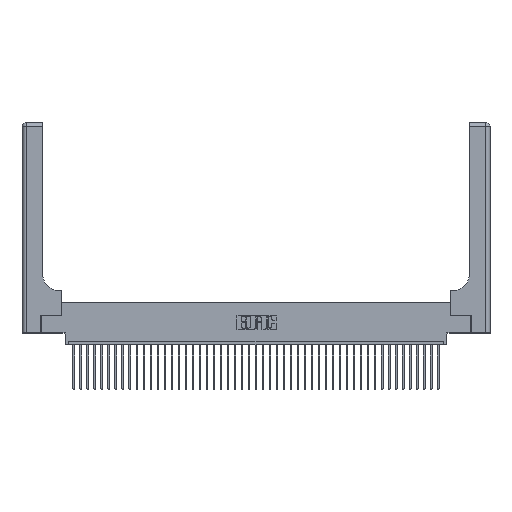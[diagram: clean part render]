
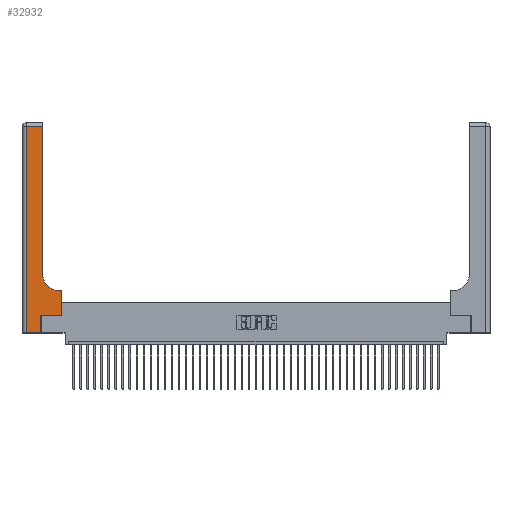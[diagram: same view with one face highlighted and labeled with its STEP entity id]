
A CAD part, top view. The second image highlights one B-rep face of the part: STEP entity #32932.
In plain terms, the highlighted planar face has unit normal (0, 0, 1).
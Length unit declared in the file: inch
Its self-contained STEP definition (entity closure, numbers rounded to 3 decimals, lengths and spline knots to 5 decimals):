
#209 = DIRECTION ( 'NONE',  ( 0., 1., 0. ) ) ;
#854 = EDGE_CURVE ( 'NONE', #1637, #6872, #2060, .T. ) ;
#1092 = CARTESIAN_POINT ( 'NONE',  ( 0., 3., 0.37 ) ) ;
#1114 = CARTESIAN_POINT ( 'NONE',  ( 0.269, 0.25, 0.37 ) ) ;
#1637 = VERTEX_POINT ( 'NONE', #42961 ) ;
#2060 = CIRCLE ( 'NONE', #29750, 0.25 ) ;
#3450 = CARTESIAN_POINT ( 'NONE',  ( 0.269, 0., 0.37 ) ) ;
#3583 = VECTOR ( 'NONE', #209, 39.37008 ) ;
#4726 = VERTEX_POINT ( 'NONE', #15478 ) ;
#5532 = CARTESIAN_POINT ( 'NONE',  ( 0.06, 0., 0.37 ) ) ;
#5651 = ORIENTED_EDGE ( 'NONE', *, *, #35412, .T. ) ;
#6872 = VERTEX_POINT ( 'NONE', #14135 ) ;
#7210 = VECTOR ( 'NONE', #16628, 39.37008 ) ;
#8408 = CARTESIAN_POINT ( 'NONE',  ( 0.5415, 0.85, 0.37 ) ) ;
#9721 = EDGE_LOOP ( 'NONE', ( #29749, #23551, #40036, #22765, #22659, #40509, #21154, #5651, #32038 ) ) ;
#10462 = LINE ( 'NONE', #3450, #27368 ) ;
#11140 = DIRECTION ( 'NONE',  ( -1., 0., 0. ) ) ;
#11336 = VERTEX_POINT ( 'NONE', #41987 ) ;
#11746 = DIRECTION ( 'NONE',  ( -1., 0., 0. ) ) ;
#12365 = CARTESIAN_POINT ( 'NONE',  ( 0.5585, 0.25, 0.37 ) ) ;
#13277 = EDGE_CURVE ( 'NONE', #34375, #34233, #33608, .T. ) ;
#13464 = CARTESIAN_POINT ( 'NONE',  ( 0., 0., 0.37 ) ) ;
#13812 = CARTESIAN_POINT ( 'NONE',  ( 0.2915, 3., 0.37 ) ) ;
#14135 = CARTESIAN_POINT ( 'NONE',  ( 0.2915, 0.85, 0.37 ) ) ;
#14227 = VECTOR ( 'NONE', #23462, 39.37008 ) ;
#15153 = VECTOR ( 'NONE', #26206, 39.37008 ) ;
#15209 = DIRECTION ( 'NONE',  ( 1., 0., 0. ) ) ;
#15478 = CARTESIAN_POINT ( 'NONE',  ( 0.2915, 2.94, 0.37 ) ) ;
#16187 = LINE ( 'NONE', #23809, #7210 ) ;
#16628 = DIRECTION ( 'NONE',  ( 1., 0., 0. ) ) ;
#18072 = VERTEX_POINT ( 'NONE', #1114 ) ;
#18288 = VECTOR ( 'NONE', #33335, 39.37008 ) ;
#18514 = CARTESIAN_POINT ( 'NONE',  ( 0.2915, 0.6, 0.37 ) ) ;
#18700 = EDGE_CURVE ( 'NONE', #6872, #4726, #23651, .T. ) ;
#20914 = CARTESIAN_POINT ( 'NONE',  ( 0.5585, 0.6, 0.37 ) ) ;
#21154 = ORIENTED_EDGE ( 'NONE', *, *, #40688, .T. ) ;
#22008 = DIRECTION ( 'NONE',  ( 0., 0., -1. ) ) ;
#22659 = ORIENTED_EDGE ( 'NONE', *, *, #35820, .T. ) ;
#22765 = ORIENTED_EDGE ( 'NONE', *, *, #34485, .T. ) ;
#23462 = DIRECTION ( 'NONE',  ( 1., 0., 0. ) ) ;
#23551 = ORIENTED_EDGE ( 'NONE', *, *, #40330, .T. ) ;
#23651 = LINE ( 'NONE', #13812, #3583 ) ;
#23809 = CARTESIAN_POINT ( 'NONE',  ( 0.269, 0.25, 0.37 ) ) ;
#24108 = VERTEX_POINT ( 'NONE', #12365 ) ;
#24414 = DIRECTION ( 'NONE',  ( 0., -1., 0. ) ) ;
#26206 = DIRECTION ( 'NONE',  ( 0., 1., 0. ) ) ;
#26987 = CARTESIAN_POINT ( 'NONE',  ( 0., 2.94, 0.37 ) ) ;
#27368 = VECTOR ( 'NONE', #40761, 39.37008 ) ;
#28361 = LINE ( 'NONE', #38571, #15153 ) ;
#28410 = CARTESIAN_POINT ( 'NONE',  ( 0.06, 3., 0.37 ) ) ;
#29533 = LINE ( 'NONE', #18514, #33225 ) ;
#29749 = ORIENTED_EDGE ( 'NONE', *, *, #18700, .T. ) ;
#29750 = AXIS2_PLACEMENT_3D ( 'NONE', #8408, #22008, #15209 ) ;
#30598 = VERTEX_POINT ( 'NONE', #20914 ) ;
#32038 = ORIENTED_EDGE ( 'NONE', *, *, #854, .T. ) ;
#32932 = ADVANCED_FACE ( 'NONE', ( #40286 ), #38118, .F. ) ;
#33225 = VECTOR ( 'NONE', #11746, 39.37008 ) ;
#33335 = DIRECTION ( 'NONE',  ( -1., 0., 0. ) ) ;
#33608 = LINE ( 'NONE', #28410, #35170 ) ;
#34233 = VERTEX_POINT ( 'NONE', #5532 ) ;
#34375 = VERTEX_POINT ( 'NONE', #42677 ) ;
#34485 = EDGE_CURVE ( 'NONE', #34233, #11336, #42220, .T. ) ;
#35170 = VECTOR ( 'NONE', #24414, 39.37008 ) ;
#35203 = DIRECTION ( 'NONE',  ( 0., 0., -1. ) ) ;
#35412 = EDGE_CURVE ( 'NONE', #30598, #1637, #29533, .T. ) ;
#35820 = EDGE_CURVE ( 'NONE', #11336, #18072, #10462, .T. ) ;
#36276 = LINE ( 'NONE', #26987, #18288 ) ;
#38118 = PLANE ( 'NONE',  #39278 ) ;
#38571 = CARTESIAN_POINT ( 'NONE',  ( 0.5585, 0.25, 0.37 ) ) ;
#39278 = AXIS2_PLACEMENT_3D ( 'NONE', #1092, #35203, #11140 ) ;
#40036 = ORIENTED_EDGE ( 'NONE', *, *, #13277, .T. ) ;
#40286 = FACE_OUTER_BOUND ( 'NONE', #9721, .T. ) ;
#40330 = EDGE_CURVE ( 'NONE', #4726, #34375, #36276, .T. ) ;
#40509 = ORIENTED_EDGE ( 'NONE', *, *, #40817, .T. ) ;
#40688 = EDGE_CURVE ( 'NONE', #24108, #30598, #28361, .T. ) ;
#40761 = DIRECTION ( 'NONE',  ( 0., 1., 0. ) ) ;
#40817 = EDGE_CURVE ( 'NONE', #18072, #24108, #16187, .T. ) ;
#41987 = CARTESIAN_POINT ( 'NONE',  ( 0.269, 0., 0.37 ) ) ;
#42220 = LINE ( 'NONE', #13464, #14227 ) ;
#42677 = CARTESIAN_POINT ( 'NONE',  ( 0.06, 2.94, 0.37 ) ) ;
#42961 = CARTESIAN_POINT ( 'NONE',  ( 0.5415, 0.6, 0.37 ) ) ;
